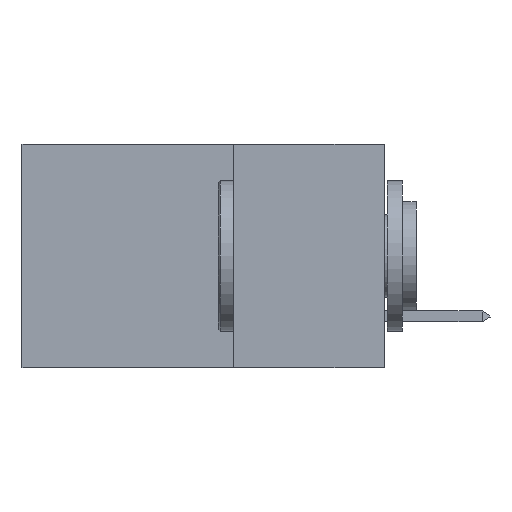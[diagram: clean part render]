
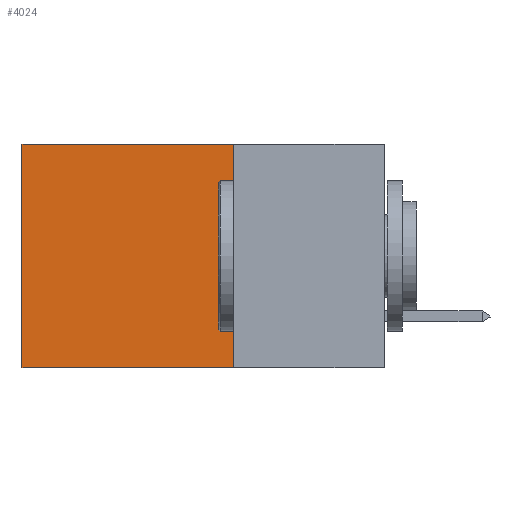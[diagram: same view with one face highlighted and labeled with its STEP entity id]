
A CAD part, left-side view. The second image highlights one B-rep face of the part: STEP entity #4024.
In plain terms, the highlighted planar face has unit normal (-1, 0, 0).
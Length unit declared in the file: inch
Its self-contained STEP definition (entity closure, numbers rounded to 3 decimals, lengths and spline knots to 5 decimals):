
#101 = CARTESIAN_POINT ( 'NONE',  ( 0.2875, 0.25, 0. ) ) ;
#289 = FACE_OUTER_BOUND ( 'NONE', #10043, .T. ) ;
#747 = CARTESIAN_POINT ( 'NONE',  ( 0.2875, 0.6, -0.37 ) ) ;
#773 = ORIENTED_EDGE ( 'NONE', *, *, #24301, .T. ) ;
#1715 = LINE ( 'NONE', #2821, #22264 ) ;
#2138 = DIRECTION ( 'NONE',  ( 0., 0., -1. ) ) ;
#2821 = CARTESIAN_POINT ( 'NONE',  ( 0.2875, 0.6, 0. ) ) ;
#4024 = ADVANCED_FACE ( 'NONE', ( #289 ), #14346, .F. ) ;
#5304 = VERTEX_POINT ( 'NONE', #747 ) ;
#5709 = CARTESIAN_POINT ( 'NONE',  ( 0.2875, 0.25, -0.37 ) ) ;
#6029 = EDGE_CURVE ( 'NONE', #15279, #5304, #24851, .T. ) ;
#6546 = VECTOR ( 'NONE', #10469, 39.37008 ) ;
#8067 = VERTEX_POINT ( 'NONE', #16127 ) ;
#8501 = ORIENTED_EDGE ( 'NONE', *, *, #16620, .T. ) ;
#8508 = VERTEX_POINT ( 'NONE', #18563 ) ;
#10043 = EDGE_LOOP ( 'NONE', ( #773, #13391, #18726, #8501 ) ) ;
#10054 = LINE ( 'NONE', #22402, #10366 ) ;
#10366 = VECTOR ( 'NONE', #14030, 39.37008 ) ;
#10469 = DIRECTION ( 'NONE',  ( 0., 0., -1. ) ) ;
#12149 = CARTESIAN_POINT ( 'NONE',  ( 0.2875, 0.25, 0. ) ) ;
#12504 = DIRECTION ( 'NONE',  ( 1., 0., 0. ) ) ;
#13391 = ORIENTED_EDGE ( 'NONE', *, *, #6029, .F. ) ;
#14030 = DIRECTION ( 'NONE',  ( 0., 1., 0. ) ) ;
#14346 = PLANE ( 'NONE',  #17759 ) ;
#15279 = VERTEX_POINT ( 'NONE', #22376 ) ;
#15701 = VECTOR ( 'NONE', #16017, 39.37008 ) ;
#16017 = DIRECTION ( 'NONE',  ( 0., 1., 0. ) ) ;
#16127 = CARTESIAN_POINT ( 'NONE',  ( 0.2875, 0.6, 0. ) ) ;
#16620 = EDGE_CURVE ( 'NONE', #8508, #8067, #10054, .T. ) ;
#16956 = DIRECTION ( 'NONE',  ( 0., 0., -1. ) ) ;
#17292 = LINE ( 'NONE', #12149, #6546 ) ;
#17445 = EDGE_CURVE ( 'NONE', #8508, #15279, #17292, .T. ) ;
#17759 = AXIS2_PLACEMENT_3D ( 'NONE', #101, #12504, #2138 ) ;
#18563 = CARTESIAN_POINT ( 'NONE',  ( 0.2875, 0.25, 0. ) ) ;
#18726 = ORIENTED_EDGE ( 'NONE', *, *, #17445, .F. ) ;
#22264 = VECTOR ( 'NONE', #16956, 39.37008 ) ;
#22376 = CARTESIAN_POINT ( 'NONE',  ( 0.2875, 0.25, -0.37 ) ) ;
#22402 = CARTESIAN_POINT ( 'NONE',  ( 0.2875, 0.25, 0. ) ) ;
#24301 = EDGE_CURVE ( 'NONE', #8067, #5304, #1715, .T. ) ;
#24851 = LINE ( 'NONE', #5709, #15701 ) ;
